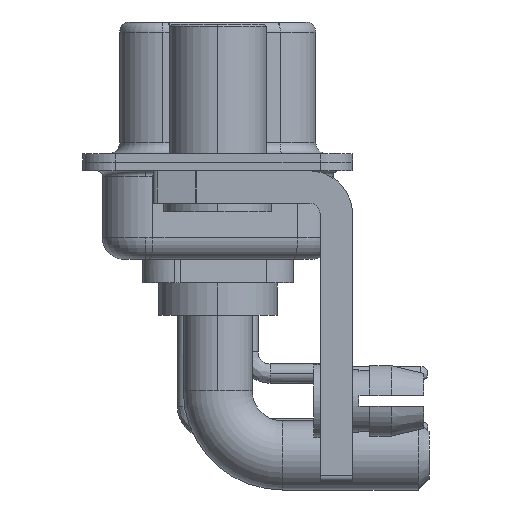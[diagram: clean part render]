
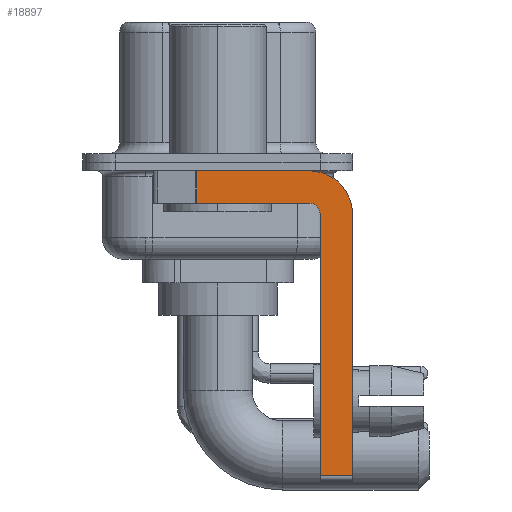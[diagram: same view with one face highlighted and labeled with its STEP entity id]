
A CAD part, left-side view. The second image highlights one B-rep face of the part: STEP entity #18897.
In plain terms, the highlighted planar face has unit normal (-1, 0, 0).
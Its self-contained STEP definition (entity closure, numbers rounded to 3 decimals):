
#818 = ORIENTED_EDGE ( 'NONE', *, *, #27611, .T. ) ;
#1054 = CIRCLE ( 'NONE', #27031, 0.5 ) ;
#2457 = CARTESIAN_POINT ( 'NONE',  ( -2.9, 0.978, -0.4 ) ) ;
#2779 = ORIENTED_EDGE ( 'NONE', *, *, #12062, .F. ) ;
#3135 = VERTEX_POINT ( 'NONE', #3324 ) ;
#3324 = CARTESIAN_POINT ( 'NONE',  ( -2.9, -4.25, -0.4 ) ) ;
#3326 = DIRECTION ( 'NONE',  ( -1., 0., 0. ) ) ;
#3375 = ORIENTED_EDGE ( 'NONE', *, *, #14092, .F. ) ;
#3845 = DIRECTION ( 'NONE',  ( 0., 0., -1. ) ) ;
#4953 = DIRECTION ( 'NONE',  ( 1., 0., 0. ) ) ;
#6456 = DIRECTION ( 'NONE',  ( 1., 0., 0. ) ) ;
#7357 = DIRECTION ( 'NONE',  ( 0., 0., -1. ) ) ;
#9302 = LINE ( 'NONE', #28082, #17910 ) ;
#9802 = AXIS2_PLACEMENT_3D ( 'NONE', #30080, #6456, #25538 ) ;
#10003 = CARTESIAN_POINT ( 'NONE',  ( -2.9, -4.75, -14.8 ) ) ;
#10348 = ORIENTED_EDGE ( 'NONE', *, *, #19548, .T. ) ;
#11107 = EDGE_CURVE ( 'NONE', #21361, #24614, #1054, .T. ) ;
#11143 = FACE_OUTER_BOUND ( 'NONE', #15878, .T. ) ;
#11524 = VECTOR ( 'NONE', #19716, 1000. ) ;
#11679 = CARTESIAN_POINT ( 'NONE',  ( -2.9, -4.25, -2.4 ) ) ;
#12062 = EDGE_CURVE ( 'NONE', #24614, #12503, #23544, .T. ) ;
#12503 = VERTEX_POINT ( 'NONE', #28471 ) ;
#12617 = ORIENTED_EDGE ( 'NONE', *, *, #11107, .F. ) ;
#13103 = CARTESIAN_POINT ( 'NONE',  ( -2.9, -6.25, -2.4 ) ) ;
#13383 = CIRCLE ( 'NONE', #25899, 2. ) ;
#13412 = CARTESIAN_POINT ( 'NONE',  ( -2.9, -4.25, -1.9 ) ) ;
#13802 = CARTESIAN_POINT ( 'NONE',  ( -2.9, -6.25, -14.55 ) ) ;
#14092 = EDGE_CURVE ( 'NONE', #28337, #14426, #20401, .T. ) ;
#14144 = CARTESIAN_POINT ( 'NONE',  ( -2.9, -4.25, -1.9 ) ) ;
#14426 = VERTEX_POINT ( 'NONE', #13802 ) ;
#15878 = EDGE_LOOP ( 'NONE', ( #27594, #10348, #2779, #12617, #16468, #818, #3375, #22493 ) ) ;
#16468 = ORIENTED_EDGE ( 'NONE', *, *, #18314, .F. ) ;
#17181 = DIRECTION ( 'NONE',  ( 0., 0., 1. ) ) ;
#17910 = VECTOR ( 'NONE', #21639, 1000. ) ;
#18314 = EDGE_CURVE ( 'NONE', #25863, #21361, #22177, .T. ) ;
#18897 = ADVANCED_FACE ( 'NONE', ( #11143 ), #30377, .F. ) ;
#19548 = EDGE_CURVE ( 'NONE', #28595, #12503, #26279, .T. ) ;
#19716 = DIRECTION ( 'NONE',  ( 0., -1., 0. ) ) ;
#20401 = LINE ( 'NONE', #29972, #29092 ) ;
#20544 = VECTOR ( 'NONE', #30891, 1000. ) ;
#20793 = VECTOR ( 'NONE', #17181, 1000. ) ;
#21361 = VERTEX_POINT ( 'NONE', #30629 ) ;
#21639 = DIRECTION ( 'NONE',  ( 0., -1., 0. ) ) ;
#21780 = VECTOR ( 'NONE', #7357, 1000. ) ;
#21880 = CARTESIAN_POINT ( 'NONE',  ( -2.9, -4.75, -14.55 ) ) ;
#21922 = DIRECTION ( 'NONE',  ( 0., 0., 1. ) ) ;
#22177 = LINE ( 'NONE', #10003, #20793 ) ;
#22493 = ORIENTED_EDGE ( 'NONE', *, *, #27222, .F. ) ;
#23544 = LINE ( 'NONE', #14144, #20544 ) ;
#23574 = DIRECTION ( 'NONE',  ( 0., 0., -1. ) ) ;
#23611 = CARTESIAN_POINT ( 'NONE',  ( -2.9, 0.978, -1.9 ) ) ;
#24614 = VERTEX_POINT ( 'NONE', #13412 ) ;
#25538 = DIRECTION ( 'NONE',  ( 0., 0., -1. ) ) ;
#25863 = VERTEX_POINT ( 'NONE', #21880 ) ;
#25899 = AXIS2_PLACEMENT_3D ( 'NONE', #11679, #4953, #23574 ) ;
#26279 = LINE ( 'NONE', #23611, #21780 ) ;
#26474 = CARTESIAN_POINT ( 'NONE',  ( -2.9, 3., -0.4 ) ) ;
#27031 = AXIS2_PLACEMENT_3D ( 'NONE', #29155, #3326, #21922 ) ;
#27222 = EDGE_CURVE ( 'NONE', #3135, #28337, #13383, .T. ) ;
#27594 = ORIENTED_EDGE ( 'NONE', *, *, #29655, .F. ) ;
#27611 = EDGE_CURVE ( 'NONE', #25863, #14426, #9302, .T. ) ;
#28082 = CARTESIAN_POINT ( 'NONE',  ( -2.9, -4.25, -14.55 ) ) ;
#28337 = VERTEX_POINT ( 'NONE', #13103 ) ;
#28471 = CARTESIAN_POINT ( 'NONE',  ( -2.9, 0.978, -1.9 ) ) ;
#28595 = VERTEX_POINT ( 'NONE', #2457 ) ;
#28824 = LINE ( 'NONE', #26474, #11524 ) ;
#29092 = VECTOR ( 'NONE', #3845, 1000. ) ;
#29155 = CARTESIAN_POINT ( 'NONE',  ( -2.9, -4.25, -2.4 ) ) ;
#29655 = EDGE_CURVE ( 'NONE', #28595, #3135, #28824, .T. ) ;
#29972 = CARTESIAN_POINT ( 'NONE',  ( -2.9, -6.25, -2.4 ) ) ;
#30080 = CARTESIAN_POINT ( 'NONE',  ( -2.9, -4.25, -2.4 ) ) ;
#30377 = PLANE ( 'NONE',  #9802 ) ;
#30629 = CARTESIAN_POINT ( 'NONE',  ( -2.9, -4.75, -2.4 ) ) ;
#30891 = DIRECTION ( 'NONE',  ( 0., 1., 0. ) ) ;
